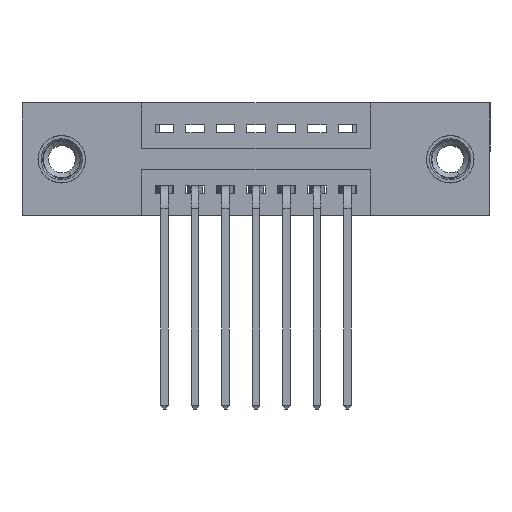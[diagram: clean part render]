
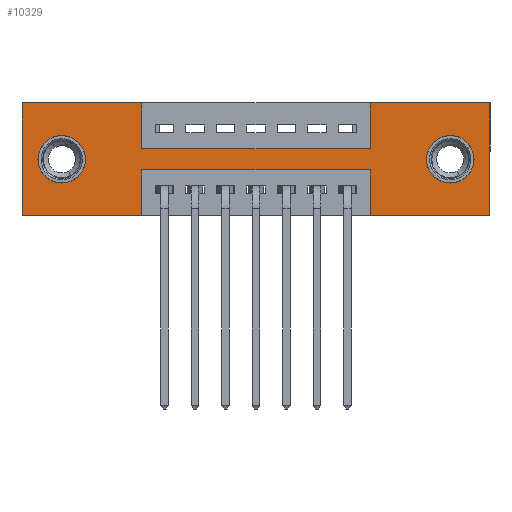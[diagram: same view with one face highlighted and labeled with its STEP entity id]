
A CAD part, front view. The second image highlights one B-rep face of the part: STEP entity #10329.
In plain terms, the highlighted planar face has unit normal (0, -1, 0).
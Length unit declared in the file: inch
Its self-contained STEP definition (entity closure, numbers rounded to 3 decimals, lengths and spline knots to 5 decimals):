
#50 = VECTOR ( 'NONE', #12509, 39.37008 ) ;
#254 = ORIENTED_EDGE ( 'NONE', *, *, #4368, .F. ) ;
#275 = VECTOR ( 'NONE', #350, 39.37008 ) ;
#350 = DIRECTION ( 'NONE',  ( -1., 0., 0. ) ) ;
#405 = LINE ( 'NONE', #7735, #50 ) ;
#672 = VERTEX_POINT ( 'NONE', #5240 ) ;
#866 = EDGE_CURVE ( 'NONE', #9011, #13226, #6952, .T. ) ;
#888 = EDGE_CURVE ( 'NONE', #907, #13167, #3889, .T. ) ;
#907 = VERTEX_POINT ( 'NONE', #2325 ) ;
#957 = CIRCLE ( 'NONE', #5307, 0.078 ) ;
#1011 = LINE ( 'NONE', #3581, #13929 ) ;
#1148 = VECTOR ( 'NONE', #12327, 39.37008 ) ;
#1241 = DIRECTION ( 'NONE',  ( 0., 0., -1. ) ) ;
#1481 = FACE_BOUND ( 'NONE', #11317, .T. ) ;
#1549 = CARTESIAN_POINT ( 'NONE',  ( 0., 0., -0.37 ) ) ;
#1618 = CARTESIAN_POINT ( 'NONE',  ( 0.13, 0., -0.263 ) ) ;
#1802 = VECTOR ( 'NONE', #5145, 39.37008 ) ;
#2097 = ORIENTED_EDGE ( 'NONE', *, *, #9990, .F. ) ;
#2213 = CARTESIAN_POINT ( 'NONE',  ( 1.535, 0., -0.37 ) ) ;
#2246 = CARTESIAN_POINT ( 'NONE',  ( 1.1425, 0., -0.37 ) ) ;
#2320 = DIRECTION ( 'NONE',  ( 0., 0., 1. ) ) ;
#2325 = CARTESIAN_POINT ( 'NONE',  ( 0.3925, 0., 0. ) ) ;
#2521 = VECTOR ( 'NONE', #6127, 39.37008 ) ;
#2692 = EDGE_CURVE ( 'NONE', #8633, #11556, #957, .T. ) ;
#3082 = DIRECTION ( 'NONE',  ( 0., 0., -1. ) ) ;
#3226 = ORIENTED_EDGE ( 'NONE', *, *, #3746, .F. ) ;
#3397 = PLANE ( 'NONE',  #10610 ) ;
#3417 = DIRECTION ( 'NONE',  ( 0., 0., 1. ) ) ;
#3467 = EDGE_CURVE ( 'NONE', #13167, #7456, #405, .T. ) ;
#3581 = CARTESIAN_POINT ( 'NONE',  ( 0., 0., 0. ) ) ;
#3746 = EDGE_CURVE ( 'NONE', #672, #9011, #10426, .T. ) ;
#3759 = LINE ( 'NONE', #10814, #1802 ) ;
#3819 = VECTOR ( 'NONE', #5405, 39.37008 ) ;
#3889 = LINE ( 'NONE', #5646, #4243 ) ;
#3916 = ORIENTED_EDGE ( 'NONE', *, *, #3467, .F. ) ;
#3991 = ORIENTED_EDGE ( 'NONE', *, *, #6963, .F. ) ;
#4086 = CARTESIAN_POINT ( 'NONE',  ( 1.405, 0., -0.185 ) ) ;
#4139 = ORIENTED_EDGE ( 'NONE', *, *, #12545, .T. ) ;
#4243 = VECTOR ( 'NONE', #7952, 39.37008 ) ;
#4368 = EDGE_CURVE ( 'NONE', #12170, #907, #3759, .T. ) ;
#4825 = CARTESIAN_POINT ( 'NONE',  ( 1.405, 0., -0.107 ) ) ;
#5145 = DIRECTION ( 'NONE',  ( 1., 0., 0. ) ) ;
#5146 = VECTOR ( 'NONE', #13148, 39.37008 ) ;
#5187 = DIRECTION ( 'NONE',  ( 0., 0., -1. ) ) ;
#5240 = CARTESIAN_POINT ( 'NONE',  ( 0.3925, 0., -0.22 ) ) ;
#5269 = CARTESIAN_POINT ( 'NONE',  ( 1.535, 0., 0. ) ) ;
#5307 = AXIS2_PLACEMENT_3D ( 'NONE', #9064, #7992, #3417 ) ;
#5389 = DIRECTION ( 'NONE',  ( -1., 0., 0. ) ) ;
#5405 = DIRECTION ( 'NONE',  ( -1., 0., 0. ) ) ;
#5550 = DIRECTION ( 'NONE',  ( 0., -1., 0. ) ) ;
#5646 = CARTESIAN_POINT ( 'NONE',  ( 0.3925, 0., 0. ) ) ;
#5813 = CARTESIAN_POINT ( 'NONE',  ( 1.405, 0., -0.185 ) ) ;
#5870 = EDGE_CURVE ( 'NONE', #7456, #9752, #14671, .T. ) ;
#6038 = DIRECTION ( 'NONE',  ( 1., 0., 0. ) ) ;
#6095 = EDGE_LOOP ( 'NONE', ( #3226, #10999, #7151, #10196, #2097, #9038, #12160, #3916, #10207, #254, #3991, #13641 ) ) ;
#6127 = DIRECTION ( 'NONE',  ( 0., 0., -1. ) ) ;
#6400 = DIRECTION ( 'NONE',  ( 0., 1., 0. ) ) ;
#6591 = CARTESIAN_POINT ( 'NONE',  ( 1.1425, 0., 0. ) ) ;
#6794 = CARTESIAN_POINT ( 'NONE',  ( 0.3925, 0., -0.37 ) ) ;
#6949 = CARTESIAN_POINT ( 'NONE',  ( 1.1425, 0., -0.15 ) ) ;
#6952 = LINE ( 'NONE', #7603, #8545 ) ;
#6963 = EDGE_CURVE ( 'NONE', #13226, #12170, #11250, .T. ) ;
#6996 = DIRECTION ( 'NONE',  ( 0., 1., 0. ) ) ;
#7151 = ORIENTED_EDGE ( 'NONE', *, *, #7723, .F. ) ;
#7456 = VERTEX_POINT ( 'NONE', #6949 ) ;
#7603 = CARTESIAN_POINT ( 'NONE',  ( 0., 0., -0.37 ) ) ;
#7646 = AXIS2_PLACEMENT_3D ( 'NONE', #12704, #6996, #2320 ) ;
#7650 = CARTESIAN_POINT ( 'NONE',  ( 1.535, 0., 0. ) ) ;
#7723 = EDGE_CURVE ( 'NONE', #14023, #14697, #14793, .T. ) ;
#7735 = CARTESIAN_POINT ( 'NONE',  ( 0.3925, 0., -0.15 ) ) ;
#7952 = DIRECTION ( 'NONE',  ( 0., 0., -1. ) ) ;
#7992 = DIRECTION ( 'NONE',  ( 0., 1., 0. ) ) ;
#8298 = EDGE_CURVE ( 'NONE', #9752, #12837, #1011, .T. ) ;
#8328 = AXIS2_PLACEMENT_3D ( 'NONE', #5813, #13824, #13879 ) ;
#8394 = ORIENTED_EDGE ( 'NONE', *, *, #2692, .T. ) ;
#8545 = VECTOR ( 'NONE', #5389, 39.37008 ) ;
#8633 = VERTEX_POINT ( 'NONE', #1618 ) ;
#8882 = DIRECTION ( 'NONE',  ( 0., 0., 1. ) ) ;
#8940 = CARTESIAN_POINT ( 'NONE',  ( 0., 0., -0.37 ) ) ;
#9011 = VERTEX_POINT ( 'NONE', #6794 ) ;
#9038 = ORIENTED_EDGE ( 'NONE', *, *, #8298, .F. ) ;
#9064 = CARTESIAN_POINT ( 'NONE',  ( 0.13, 0., -0.185 ) ) ;
#9177 = FACE_BOUND ( 'NONE', #12604, .T. ) ;
#9380 = CARTESIAN_POINT ( 'NONE',  ( 0.3925, 0., -0.37 ) ) ;
#9398 = ORIENTED_EDGE ( 'NONE', *, *, #9899, .T. ) ;
#9448 = EDGE_CURVE ( 'NONE', #13080, #14023, #13888, .T. ) ;
#9721 = EDGE_CURVE ( 'NONE', #14697, #672, #11366, .T. ) ;
#9752 = VERTEX_POINT ( 'NONE', #14722 ) ;
#9767 = CARTESIAN_POINT ( 'NONE',  ( 0.13, 0., -0.107 ) ) ;
#9899 = EDGE_CURVE ( 'NONE', #10253, #13705, #13158, .T. ) ;
#9990 = EDGE_CURVE ( 'NONE', #12837, #13080, #11173, .T. ) ;
#10192 = ORIENTED_EDGE ( 'NONE', *, *, #13583, .T. ) ;
#10196 = ORIENTED_EDGE ( 'NONE', *, *, #9448, .F. ) ;
#10205 = CIRCLE ( 'NONE', #7646, 0.078 ) ;
#10207 = ORIENTED_EDGE ( 'NONE', *, *, #888, .F. ) ;
#10253 = VERTEX_POINT ( 'NONE', #4825 ) ;
#10329 = ADVANCED_FACE ( 'NONE', ( #9177, #1481, #10450 ), #3397, .T. ) ;
#10426 = LINE ( 'NONE', #9380, #2521 ) ;
#10450 = FACE_OUTER_BOUND ( 'NONE', #6095, .T. ) ;
#10610 = AXIS2_PLACEMENT_3D ( 'NONE', #8940, #5550, #1241 ) ;
#10814 = CARTESIAN_POINT ( 'NONE',  ( 0., 0., 0. ) ) ;
#10818 = CARTESIAN_POINT ( 'NONE',  ( 1.405, 0., -0.263 ) ) ;
#10846 = CARTESIAN_POINT ( 'NONE',  ( 0., 0., 0. ) ) ;
#10900 = AXIS2_PLACEMENT_3D ( 'NONE', #4086, #6400, #5187 ) ;
#10987 = VECTOR ( 'NONE', #3082, 39.37008 ) ;
#10999 = ORIENTED_EDGE ( 'NONE', *, *, #9721, .F. ) ;
#11173 = LINE ( 'NONE', #7650, #10987 ) ;
#11207 = CARTESIAN_POINT ( 'NONE',  ( 0., 0., 0. ) ) ;
#11250 = LINE ( 'NONE', #10846, #5146 ) ;
#11317 = EDGE_LOOP ( 'NONE', ( #4139, #8394 ) ) ;
#11366 = LINE ( 'NONE', #12413, #3819 ) ;
#11556 = VERTEX_POINT ( 'NONE', #9767 ) ;
#11650 = VECTOR ( 'NONE', #8882, 39.37008 ) ;
#12160 = ORIENTED_EDGE ( 'NONE', *, *, #5870, .F. ) ;
#12170 = VERTEX_POINT ( 'NONE', #11207 ) ;
#12327 = DIRECTION ( 'NONE',  ( 0., 0., 1. ) ) ;
#12413 = CARTESIAN_POINT ( 'NONE',  ( 0.3925, 0., -0.22 ) ) ;
#12509 = DIRECTION ( 'NONE',  ( 1., 0., 0. ) ) ;
#12545 = EDGE_CURVE ( 'NONE', #11556, #8633, #10205, .T. ) ;
#12604 = EDGE_LOOP ( 'NONE', ( #9398, #10192 ) ) ;
#12704 = CARTESIAN_POINT ( 'NONE',  ( 0.13, 0., -0.185 ) ) ;
#12786 = CARTESIAN_POINT ( 'NONE',  ( 0.3925, 0., -0.15 ) ) ;
#12837 = VERTEX_POINT ( 'NONE', #5269 ) ;
#13080 = VERTEX_POINT ( 'NONE', #2213 ) ;
#13148 = DIRECTION ( 'NONE',  ( 0., 0., 1. ) ) ;
#13158 = CIRCLE ( 'NONE', #10900, 0.078 ) ;
#13167 = VERTEX_POINT ( 'NONE', #12786 ) ;
#13226 = VERTEX_POINT ( 'NONE', #1549 ) ;
#13583 = EDGE_CURVE ( 'NONE', #13705, #10253, #14471, .T. ) ;
#13641 = ORIENTED_EDGE ( 'NONE', *, *, #866, .F. ) ;
#13705 = VERTEX_POINT ( 'NONE', #10818 ) ;
#13752 = CARTESIAN_POINT ( 'NONE',  ( 1.1425, 0., -0.22 ) ) ;
#13824 = DIRECTION ( 'NONE',  ( 0., 1., 0. ) ) ;
#13879 = DIRECTION ( 'NONE',  ( 0., 0., -1. ) ) ;
#13888 = LINE ( 'NONE', #13930, #275 ) ;
#13929 = VECTOR ( 'NONE', #6038, 39.37008 ) ;
#13930 = CARTESIAN_POINT ( 'NONE',  ( 0., 0., -0.37 ) ) ;
#14023 = VERTEX_POINT ( 'NONE', #2246 ) ;
#14471 = CIRCLE ( 'NONE', #8328, 0.078 ) ;
#14576 = CARTESIAN_POINT ( 'NONE',  ( 1.1425, 0., -0.37 ) ) ;
#14671 = LINE ( 'NONE', #6591, #11650 ) ;
#14697 = VERTEX_POINT ( 'NONE', #13752 ) ;
#14722 = CARTESIAN_POINT ( 'NONE',  ( 1.1425, 0., 0. ) ) ;
#14793 = LINE ( 'NONE', #14576, #1148 ) ;
